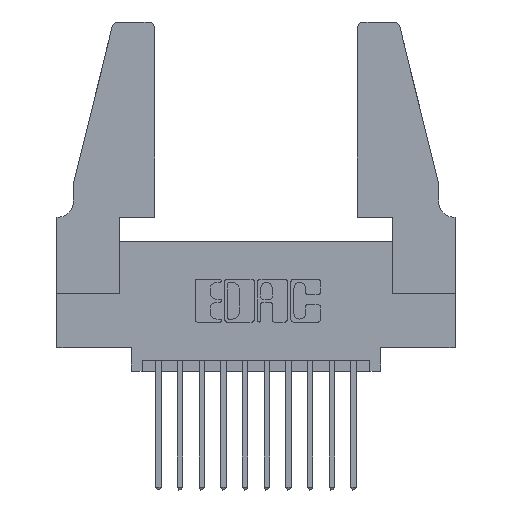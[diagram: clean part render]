
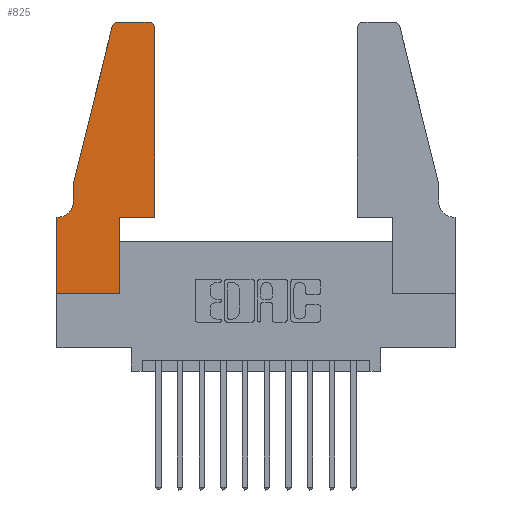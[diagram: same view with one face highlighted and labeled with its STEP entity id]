
A CAD part, top view. The second image highlights one B-rep face of the part: STEP entity #825.
In plain terms, the highlighted planar face has unit normal (0, 0, 1).
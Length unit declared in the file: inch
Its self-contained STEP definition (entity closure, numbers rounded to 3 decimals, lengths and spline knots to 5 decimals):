
#26 = EDGE_CURVE ( 'NONE', #12914, #10883, #717, .T. ) ;
#74 = VECTOR ( 'NONE', #3572, 39.37008 ) ;
#384 = LINE ( 'NONE', #9853, #8992 ) ;
#394 = AXIS2_PLACEMENT_3D ( 'NONE', #8844, #13338, #945 ) ;
#449 = ORIENTED_EDGE ( 'NONE', *, *, #11329, .T. ) ;
#717 = LINE ( 'NONE', #11187, #14358 ) ;
#825 = ADVANCED_FACE ( 'NONE', ( #9755 ), #5963, .T. ) ;
#868 = ORIENTED_EDGE ( 'NONE', *, *, #11066, .T. ) ;
#900 = VERTEX_POINT ( 'NONE', #5118 ) ;
#913 = LINE ( 'NONE', #12455, #5874 ) ;
#945 = DIRECTION ( 'NONE',  ( -1., 0., 0. ) ) ;
#1016 = EDGE_CURVE ( 'NONE', #10883, #4206, #12534, .T. ) ;
#1215 = VERTEX_POINT ( 'NONE', #6718 ) ;
#1473 = ORIENTED_EDGE ( 'NONE', *, *, #3669, .T. ) ;
#1795 = CARTESIAN_POINT ( 'NONE',  ( 0.0755, 0.5, 0.37 ) ) ;
#1818 = EDGE_CURVE ( 'NONE', #4206, #1215, #9553, .T. ) ;
#1832 = DIRECTION ( 'NONE',  ( 0., 0., 1. ) ) ;
#1884 = DIRECTION ( 'NONE',  ( 1., 0., 0. ) ) ;
#2253 = CARTESIAN_POINT ( 'NONE',  ( 0.4505, 1.22, 0.37 ) ) ;
#2323 = DIRECTION ( 'NONE',  ( -0.239, -0.971, 0. ) ) ;
#2510 = VECTOR ( 'NONE', #3748, 39.37008 ) ;
#2955 = CARTESIAN_POINT ( 'NONE',  ( 0., 0.35, 0.37 ) ) ;
#3008 = VECTOR ( 'NONE', #3060, 39.37008 ) ;
#3060 = DIRECTION ( 'NONE',  ( -1., 0., 0. ) ) ;
#3466 = ORIENTED_EDGE ( 'NONE', *, *, #3725, .T. ) ;
#3475 = DIRECTION ( 'NONE',  ( 1., 0., 0. ) ) ;
#3572 = DIRECTION ( 'NONE',  ( 0., 1., 0. ) ) ;
#3669 = EDGE_CURVE ( 'NONE', #12452, #8833, #6416, .T. ) ;
#3725 = EDGE_CURVE ( 'NONE', #12170, #11300, #384, .T. ) ;
#3748 = DIRECTION ( 'NONE',  ( 0., -1., 0. ) ) ;
#3853 = CARTESIAN_POINT ( 'NONE',  ( 0., 0.35, 0.37 ) ) ;
#4206 = VERTEX_POINT ( 'NONE', #7663 ) ;
#4426 = DIRECTION ( 'NONE',  ( 0., 1., 0. ) ) ;
#4497 = ORIENTED_EDGE ( 'NONE', *, *, #6095, .T. ) ;
#4609 = DIRECTION ( 'NONE',  ( 0., 0., 1. ) ) ;
#4968 = CARTESIAN_POINT ( 'NONE',  ( 0.2865, 0., 0.37 ) ) ;
#4969 = EDGE_CURVE ( 'NONE', #6925, #6131, #9801, .T. ) ;
#5050 = EDGE_CURVE ( 'NONE', #8833, #6925, #11574, .T. ) ;
#5118 = CARTESIAN_POINT ( 'NONE',  ( 0.2865, 0.35, 0.37 ) ) ;
#5171 = ORIENTED_EDGE ( 'NONE', *, *, #13049, .T. ) ;
#5288 = VECTOR ( 'NONE', #7331, 39.37008 ) ;
#5479 = CARTESIAN_POINT ( 'NONE',  ( 0.0755, 0.35, 0.37 ) ) ;
#5640 = DIRECTION ( 'NONE',  ( 1., 0., 0. ) ) ;
#5874 = VECTOR ( 'NONE', #5640, 39.37008 ) ;
#5963 = PLANE ( 'NONE',  #9204 ) ;
#6095 = EDGE_CURVE ( 'NONE', #900, #12170, #11548, .T. ) ;
#6112 = LINE ( 'NONE', #10401, #74 ) ;
#6131 = VERTEX_POINT ( 'NONE', #7619 ) ;
#6339 = DIRECTION ( 'NONE',  ( 0., -1., 0. ) ) ;
#6416 = CIRCLE ( 'NONE', #394, 0.07 ) ;
#6588 = LINE ( 'NONE', #1795, #2510 ) ;
#6718 = CARTESIAN_POINT ( 'NONE',  ( 0.0755, 0.5, 0.37 ) ) ;
#6925 = VERTEX_POINT ( 'NONE', #2955 ) ;
#6946 = CARTESIAN_POINT ( 'NONE',  ( 0.0055, 0.35, 0.37 ) ) ;
#7277 = DIRECTION ( 'NONE',  ( 0., 0., 1. ) ) ;
#7331 = DIRECTION ( 'NONE',  ( 1., 0., 0. ) ) ;
#7380 = CARTESIAN_POINT ( 'NONE',  ( 0.4505, 0.35, 0.37 ) ) ;
#7537 = CARTESIAN_POINT ( 'NONE',  ( 0., 0., 0.37 ) ) ;
#7619 = CARTESIAN_POINT ( 'NONE',  ( 0., 0., 0.37 ) ) ;
#7663 = CARTESIAN_POINT ( 'NONE',  ( 0.25487, 1.22718, 0.37 ) ) ;
#8396 = CARTESIAN_POINT ( 'NONE',  ( 0.4505, 0.35, 0.37 ) ) ;
#8433 = DIRECTION ( 'NONE',  ( 1., 0., 0. ) ) ;
#8755 = ORIENTED_EDGE ( 'NONE', *, *, #4969, .T. ) ;
#8833 = VERTEX_POINT ( 'NONE', #6946 ) ;
#8844 = CARTESIAN_POINT ( 'NONE',  ( 0.0055, 0.42, 0.37 ) ) ;
#8917 = ORIENTED_EDGE ( 'NONE', *, *, #1016, .T. ) ;
#8992 = VECTOR ( 'NONE', #4426, 39.37008 ) ;
#9120 = VECTOR ( 'NONE', #6339, 39.37008 ) ;
#9204 = AXIS2_PLACEMENT_3D ( 'NONE', #3853, #7277, #8433 ) ;
#9211 = ORIENTED_EDGE ( 'NONE', *, *, #1818, .T. ) ;
#9508 = EDGE_CURVE ( 'NONE', #9848, #900, #6112, .T. ) ;
#9553 = LINE ( 'NONE', #13596, #13207 ) ;
#9755 = FACE_OUTER_BOUND ( 'NONE', #10549, .T. ) ;
#9801 = LINE ( 'NONE', #7537, #9120 ) ;
#9848 = VERTEX_POINT ( 'NONE', #4968 ) ;
#9853 = CARTESIAN_POINT ( 'NONE',  ( 0.4505, 0.35, 0.37 ) ) ;
#10072 = CARTESIAN_POINT ( 'NONE',  ( 0.4205, 1.22, 0.37 ) ) ;
#10274 = ORIENTED_EDGE ( 'NONE', *, *, #5050, .T. ) ;
#10401 = CARTESIAN_POINT ( 'NONE',  ( 0.2865, 0.35, 0.37 ) ) ;
#10549 = EDGE_LOOP ( 'NONE', ( #11755, #8917, #9211, #868, #1473, #10274, #8755, #449, #10750, #4497, #3466, #5171 ) ) ;
#10750 = ORIENTED_EDGE ( 'NONE', *, *, #9508, .T. ) ;
#10883 = VERTEX_POINT ( 'NONE', #10951 ) ;
#10951 = CARTESIAN_POINT ( 'NONE',  ( 0.284, 1.25, 0.37 ) ) ;
#11066 = EDGE_CURVE ( 'NONE', #1215, #12452, #6588, .T. ) ;
#11082 = DIRECTION ( 'NONE',  ( -1., 0., 0. ) ) ;
#11145 = AXIS2_PLACEMENT_3D ( 'NONE', #12011, #1832, #1884 ) ;
#11187 = CARTESIAN_POINT ( 'NONE',  ( 0.2605, 1.25, 0.37 ) ) ;
#11300 = VERTEX_POINT ( 'NONE', #2253 ) ;
#11329 = EDGE_CURVE ( 'NONE', #6131, #9848, #913, .T. ) ;
#11542 = CIRCLE ( 'NONE', #13393, 0.03 ) ;
#11548 = LINE ( 'NONE', #7380, #5288 ) ;
#11574 = LINE ( 'NONE', #5479, #3008 ) ;
#11755 = ORIENTED_EDGE ( 'NONE', *, *, #26, .T. ) ;
#12011 = CARTESIAN_POINT ( 'NONE',  ( 0.284, 1.22, 0.37 ) ) ;
#12141 = CARTESIAN_POINT ( 'NONE',  ( 0.4205, 1.25, 0.37 ) ) ;
#12170 = VERTEX_POINT ( 'NONE', #8396 ) ;
#12239 = CARTESIAN_POINT ( 'NONE',  ( 0.0755, 0.42, 0.37 ) ) ;
#12452 = VERTEX_POINT ( 'NONE', #12239 ) ;
#12455 = CARTESIAN_POINT ( 'NONE',  ( 0., 0., 0.37 ) ) ;
#12534 = CIRCLE ( 'NONE', #11145, 0.03 ) ;
#12914 = VERTEX_POINT ( 'NONE', #12141 ) ;
#13049 = EDGE_CURVE ( 'NONE', #11300, #12914, #11542, .T. ) ;
#13207 = VECTOR ( 'NONE', #2323, 39.37008 ) ;
#13338 = DIRECTION ( 'NONE',  ( 0., 0., -1. ) ) ;
#13393 = AXIS2_PLACEMENT_3D ( 'NONE', #10072, #4609, #3475 ) ;
#13596 = CARTESIAN_POINT ( 'NONE',  ( 0.0755, 0.5, 0.37 ) ) ;
#14358 = VECTOR ( 'NONE', #11082, 39.37008 ) ;
